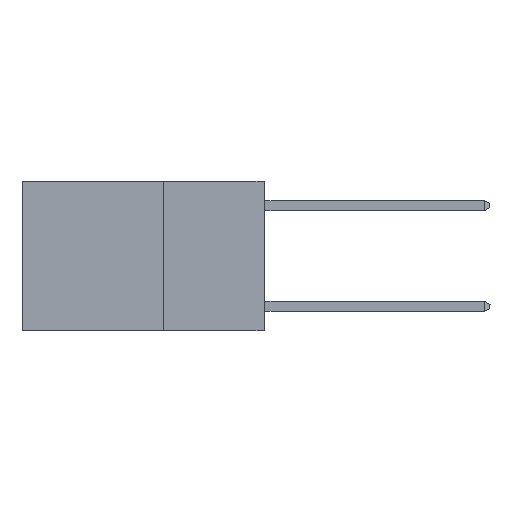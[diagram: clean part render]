
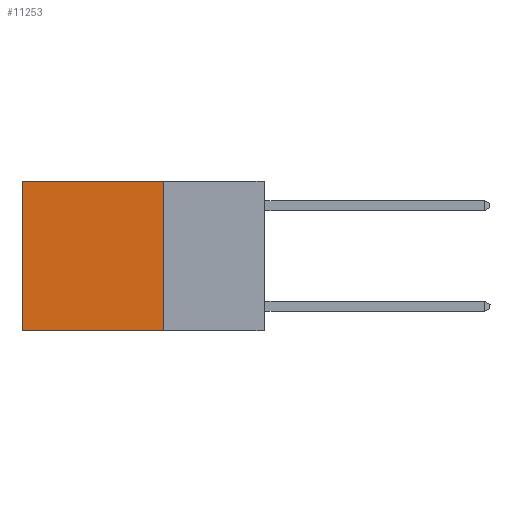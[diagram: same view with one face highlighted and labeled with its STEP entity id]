
A CAD part, left-side view. The second image highlights one B-rep face of the part: STEP entity #11253.
In plain terms, the highlighted planar face has unit normal (-1, 0, 0).
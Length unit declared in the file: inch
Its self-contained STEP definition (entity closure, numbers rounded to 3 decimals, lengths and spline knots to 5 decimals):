
#337 = DIRECTION ( 'NONE',  ( 0., 0., -1. ) ) ;
#2236 = VERTEX_POINT ( 'NONE', #15534 ) ;
#3431 = CARTESIAN_POINT ( 'NONE',  ( 0.2625, 0.6, 0. ) ) ;
#3473 = DIRECTION ( 'NONE',  ( 0., 1., 0. ) ) ;
#3898 = CARTESIAN_POINT ( 'NONE',  ( 0.2625, 0.25, 0. ) ) ;
#4203 = VECTOR ( 'NONE', #337, 39.37008 ) ;
#5428 = CARTESIAN_POINT ( 'NONE',  ( 0.2625, 0.6, 0. ) ) ;
#5990 = CARTESIAN_POINT ( 'NONE',  ( 0.2625, 0.25, 0. ) ) ;
#6092 = AXIS2_PLACEMENT_3D ( 'NONE', #11850, #19465, #13591 ) ;
#6161 = LINE ( 'NONE', #9316, #13781 ) ;
#6634 = FACE_OUTER_BOUND ( 'NONE', #15119, .T. ) ;
#6735 = VERTEX_POINT ( 'NONE', #5428 ) ;
#6801 = ORIENTED_EDGE ( 'NONE', *, *, #14314, .T. ) ;
#8908 = LINE ( 'NONE', #5990, #15087 ) ;
#9316 = CARTESIAN_POINT ( 'NONE',  ( 0.2625, 0.25, -0.37 ) ) ;
#10883 = EDGE_CURVE ( 'NONE', #12196, #6735, #12758, .T. ) ;
#11253 = ADVANCED_FACE ( 'NONE', ( #6634 ), #11978, .F. ) ;
#11577 = ORIENTED_EDGE ( 'NONE', *, *, #16316, .F. ) ;
#11657 = DIRECTION ( 'NONE',  ( 0., 1., 0. ) ) ;
#11850 = CARTESIAN_POINT ( 'NONE',  ( 0.2625, 0.25, 0. ) ) ;
#11978 = PLANE ( 'NONE',  #6092 ) ;
#12196 = VERTEX_POINT ( 'NONE', #19600 ) ;
#12758 = LINE ( 'NONE', #3898, #17324 ) ;
#13014 = EDGE_CURVE ( 'NONE', #18332, #2236, #6161, .T. ) ;
#13268 = ORIENTED_EDGE ( 'NONE', *, *, #10883, .T. ) ;
#13591 = DIRECTION ( 'NONE',  ( 0., 0., -1. ) ) ;
#13781 = VECTOR ( 'NONE', #3473, 39.37008 ) ;
#14314 = EDGE_CURVE ( 'NONE', #6735, #2236, #18027, .T. ) ;
#15087 = VECTOR ( 'NONE', #19660, 39.37008 ) ;
#15119 = EDGE_LOOP ( 'NONE', ( #6801, #16388, #11577, #13268 ) ) ;
#15534 = CARTESIAN_POINT ( 'NONE',  ( 0.2625, 0.6, -0.37 ) ) ;
#16316 = EDGE_CURVE ( 'NONE', #12196, #18332, #8908, .T. ) ;
#16388 = ORIENTED_EDGE ( 'NONE', *, *, #13014, .F. ) ;
#16609 = CARTESIAN_POINT ( 'NONE',  ( 0.2625, 0.25, -0.37 ) ) ;
#17324 = VECTOR ( 'NONE', #11657, 39.37008 ) ;
#18027 = LINE ( 'NONE', #3431, #4203 ) ;
#18332 = VERTEX_POINT ( 'NONE', #16609 ) ;
#19465 = DIRECTION ( 'NONE',  ( 1., 0., 0. ) ) ;
#19600 = CARTESIAN_POINT ( 'NONE',  ( 0.2625, 0.25, 0. ) ) ;
#19660 = DIRECTION ( 'NONE',  ( 0., 0., -1. ) ) ;
